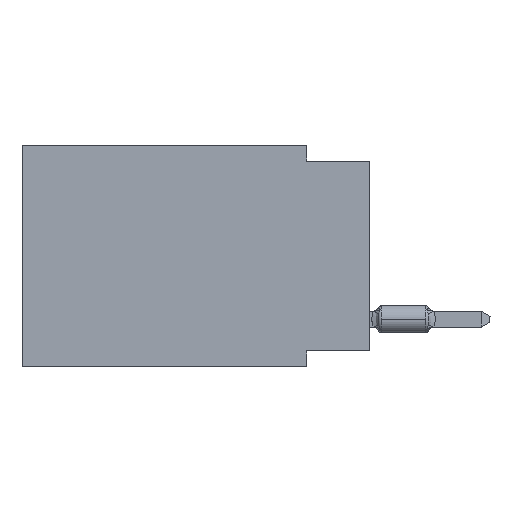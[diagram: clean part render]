
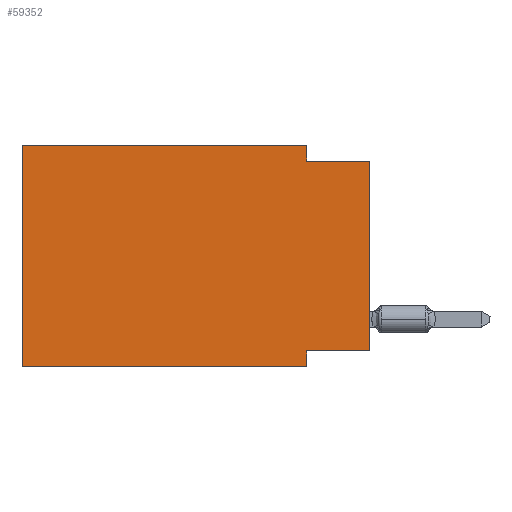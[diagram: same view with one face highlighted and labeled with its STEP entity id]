
A CAD part, left-side view. The second image highlights one B-rep face of the part: STEP entity #59352.
In plain terms, the highlighted planar face has unit normal (-1, 0, 0).
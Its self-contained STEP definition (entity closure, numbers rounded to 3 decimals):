
#72 = VERTEX_POINT ( 'NONE', #59888 ) ;
#2246 = LINE ( 'NONE', #63233, #91175 ) ;
#2752 = DIRECTION ( 'NONE',  ( 0., -1., 0. ) ) ;
#2911 = ORIENTED_EDGE ( 'NONE', *, *, #17285, .F. ) ;
#4834 = CARTESIAN_POINT ( 'NONE',  ( 0., 13.97, 0. ) ) ;
#4997 = CARTESIAN_POINT ( 'NONE',  ( 0., 0., -8.255 ) ) ;
#6065 = EDGE_CURVE ( 'NONE', #72, #10485, #92419, .T. ) ;
#7362 = EDGE_LOOP ( 'NONE', ( #59420, #57132, #2911, #64249, #76882, #68175, #45549, #28123 ) ) ;
#7577 = VECTOR ( 'NONE', #35246, 1000. ) ;
#10485 = VERTEX_POINT ( 'NONE', #57409 ) ;
#11355 = CARTESIAN_POINT ( 'NONE',  ( 0., 0., -0.635 ) ) ;
#14030 = CARTESIAN_POINT ( 'NONE',  ( 0., 13.97, 0. ) ) ;
#17285 = EDGE_CURVE ( 'NONE', #80398, #18729, #62716, .T. ) ;
#18519 = DIRECTION ( 'NONE',  ( 0., 0., -1. ) ) ;
#18729 = VERTEX_POINT ( 'NONE', #93628 ) ;
#19185 = PLANE ( 'NONE',  #39552 ) ;
#19668 = FACE_OUTER_BOUND ( 'NONE', #7362, .T. ) ;
#20792 = EDGE_CURVE ( 'NONE', #72, #72019, #44297, .T. ) ;
#21353 = VERTEX_POINT ( 'NONE', #57351 ) ;
#21719 = VECTOR ( 'NONE', #18519, 1000. ) ;
#25061 = CARTESIAN_POINT ( 'NONE',  ( 0., 2.54, 0. ) ) ;
#25349 = EDGE_CURVE ( 'NONE', #72019, #80398, #2246, .T. ) ;
#28123 = ORIENTED_EDGE ( 'NONE', *, *, #69182, .F. ) ;
#28555 = VERTEX_POINT ( 'NONE', #40921 ) ;
#30361 = VECTOR ( 'NONE', #68055, 1000. ) ;
#34555 = CARTESIAN_POINT ( 'NONE',  ( 0., 13.97, 0. ) ) ;
#35246 = DIRECTION ( 'NONE',  ( 0., 1., 0. ) ) ;
#37482 = CARTESIAN_POINT ( 'NONE',  ( 0., 0., 0. ) ) ;
#39361 = CARTESIAN_POINT ( 'NONE',  ( 0., 13.97, -8.89 ) ) ;
#39552 = AXIS2_PLACEMENT_3D ( 'NONE', #34555, #71746, #95077 ) ;
#39851 = CARTESIAN_POINT ( 'NONE',  ( 0., 2.54, -8.89 ) ) ;
#40921 = CARTESIAN_POINT ( 'NONE',  ( 0., 0., -8.255 ) ) ;
#41808 = CARTESIAN_POINT ( 'NONE',  ( 0., 2.54, 0. ) ) ;
#44297 = LINE ( 'NONE', #14030, #30361 ) ;
#44404 = VECTOR ( 'NONE', #92494, 1000. ) ;
#45549 = ORIENTED_EDGE ( 'NONE', *, *, #61620, .F. ) ;
#47469 = EDGE_CURVE ( 'NONE', #18729, #81415, #49056, .T. ) ;
#48279 = DIRECTION ( 'NONE',  ( 0., -1., 0. ) ) ;
#48778 = LINE ( 'NONE', #39851, #21719 ) ;
#49056 = LINE ( 'NONE', #11355, #71305 ) ;
#57132 = ORIENTED_EDGE ( 'NONE', *, *, #47469, .F. ) ;
#57351 = CARTESIAN_POINT ( 'NONE',  ( 0., 2.54, -8.255 ) ) ;
#57409 = CARTESIAN_POINT ( 'NONE',  ( 0., 2.54, -8.89 ) ) ;
#59352 = ADVANCED_FACE ( 'NONE', ( #19668 ), #19185, .F. ) ;
#59420 = ORIENTED_EDGE ( 'NONE', *, *, #89078, .T. ) ;
#59888 = CARTESIAN_POINT ( 'NONE',  ( 0., 13.97, -8.89 ) ) ;
#61620 = EDGE_CURVE ( 'NONE', #21353, #10485, #48778, .T. ) ;
#62716 = LINE ( 'NONE', #25061, #44404 ) ;
#63233 = CARTESIAN_POINT ( 'NONE',  ( 0., 13.97, 0. ) ) ;
#64196 = VECTOR ( 'NONE', #97507, 1000. ) ;
#64249 = ORIENTED_EDGE ( 'NONE', *, *, #25349, .F. ) ;
#65981 = LINE ( 'NONE', #4997, #7577 ) ;
#68055 = DIRECTION ( 'NONE',  ( 0., 0., 1. ) ) ;
#68175 = ORIENTED_EDGE ( 'NONE', *, *, #6065, .T. ) ;
#69182 = EDGE_CURVE ( 'NONE', #28555, #21353, #65981, .T. ) ;
#71305 = VECTOR ( 'NONE', #85264, 1000. ) ;
#71746 = DIRECTION ( 'NONE',  ( 1., 0., 0. ) ) ;
#72019 = VERTEX_POINT ( 'NONE', #4834 ) ;
#72995 = CARTESIAN_POINT ( 'NONE',  ( 0., 0., -0.635 ) ) ;
#76882 = ORIENTED_EDGE ( 'NONE', *, *, #20792, .F. ) ;
#80398 = VERTEX_POINT ( 'NONE', #41808 ) ;
#81415 = VERTEX_POINT ( 'NONE', #72995 ) ;
#85264 = DIRECTION ( 'NONE',  ( 0., -1., 0. ) ) ;
#89078 = EDGE_CURVE ( 'NONE', #28555, #81415, #90073, .T. ) ;
#90073 = LINE ( 'NONE', #37482, #64196 ) ;
#91175 = VECTOR ( 'NONE', #2752, 1000. ) ;
#92419 = LINE ( 'NONE', #39361, #93398 ) ;
#92494 = DIRECTION ( 'NONE',  ( 0., 0., -1. ) ) ;
#93398 = VECTOR ( 'NONE', #48279, 1000. ) ;
#93628 = CARTESIAN_POINT ( 'NONE',  ( 0., 2.54, -0.635 ) ) ;
#95077 = DIRECTION ( 'NONE',  ( 0., 0., -1. ) ) ;
#97507 = DIRECTION ( 'NONE',  ( 0., 0., 1. ) ) ;
